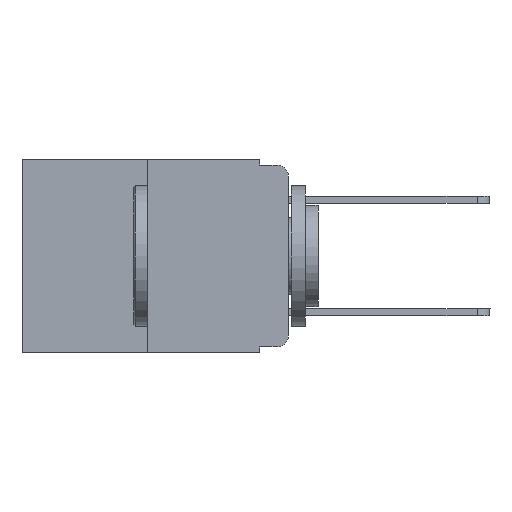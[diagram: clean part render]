
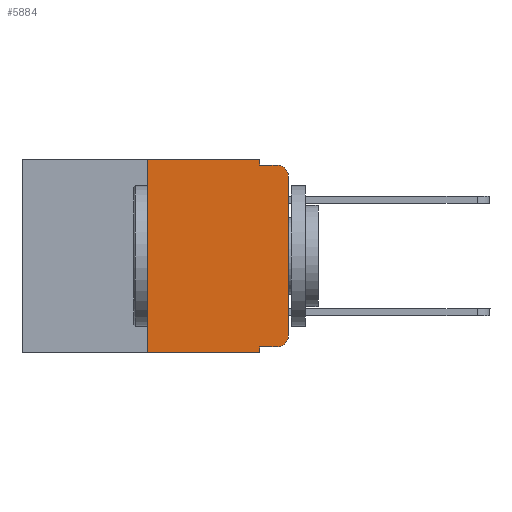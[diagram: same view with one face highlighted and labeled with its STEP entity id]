
A CAD part, left-side view. The second image highlights one B-rep face of the part: STEP entity #5884.
In plain terms, the highlighted planar face has unit normal (-1, 0, 0).
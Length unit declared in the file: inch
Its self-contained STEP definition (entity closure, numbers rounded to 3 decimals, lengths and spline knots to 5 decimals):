
#349 = CARTESIAN_POINT ( 'NONE',  ( 0., 0.051, -0.333 ) ) ;
#657 = DIRECTION ( 'NONE',  ( 0., -1., 0. ) ) ;
#759 = CARTESIAN_POINT ( 'NONE',  ( 0., 0.051, 0. ) ) ;
#1233 = LINE ( 'NONE', #5460, #2281 ) ;
#1268 = CARTESIAN_POINT ( 'NONE',  ( 0., 0.473, 0. ) ) ;
#1450 = LINE ( 'NONE', #349, #11938 ) ;
#1746 = CARTESIAN_POINT ( 'NONE',  ( 0., 0.051, -0.01 ) ) ;
#2281 = VECTOR ( 'NONE', #13563, 39.37008 ) ;
#2683 = ORIENTED_EDGE ( 'NONE', *, *, #13855, .F. ) ;
#2717 = EDGE_CURVE ( 'NONE', #15281, #13581, #4528, .T. ) ;
#2889 = DIRECTION ( 'NONE',  ( 1., 0., 0. ) ) ;
#2960 = DIRECTION ( 'NONE',  ( 0., -1., 0. ) ) ;
#2986 = VERTEX_POINT ( 'NONE', #11267 ) ;
#2997 = EDGE_CURVE ( 'NONE', #15556, #3769, #9913, .T. ) ;
#3769 = VERTEX_POINT ( 'NONE', #13083 ) ;
#3792 = DIRECTION ( 'NONE',  ( -1., 0., 0. ) ) ;
#4029 = EDGE_CURVE ( 'NONE', #12999, #17252, #9879, .T. ) ;
#4117 = DIRECTION ( 'NONE',  ( 0., 0., -1. ) ) ;
#4300 = VECTOR ( 'NONE', #4349, 39.37008 ) ;
#4349 = DIRECTION ( 'NONE',  ( 0., -1., 0. ) ) ;
#4528 = LINE ( 'NONE', #1268, #10793 ) ;
#4591 = ORIENTED_EDGE ( 'NONE', *, *, #5762, .T. ) ;
#4881 = CARTESIAN_POINT ( 'NONE',  ( 0., 0.02, -0.333 ) ) ;
#5241 = EDGE_CURVE ( 'NONE', #2986, #13518, #1450, .T. ) ;
#5460 = CARTESIAN_POINT ( 'NONE',  ( 0., 0.25, 0. ) ) ;
#5762 = EDGE_CURVE ( 'NONE', #13518, #15556, #9610, .T. ) ;
#5884 = ADVANCED_FACE ( 'NONE', ( #13840 ), #8219, .F. ) ;
#6357 = DIRECTION ( 'NONE',  ( 0., 0., -1. ) ) ;
#6586 = ORIENTED_EDGE ( 'NONE', *, *, #2717, .F. ) ;
#6809 = EDGE_CURVE ( 'NONE', #2986, #10002, #9360, .T. ) ;
#6993 = VECTOR ( 'NONE', #6357, 39.37008 ) ;
#7053 = CARTESIAN_POINT ( 'NONE',  ( 0., 0.02, -0.313 ) ) ;
#7105 = DIRECTION ( 'NONE',  ( 0., 0., 1. ) ) ;
#7836 = ORIENTED_EDGE ( 'NONE', *, *, #2997, .T. ) ;
#7860 = AXIS2_PLACEMENT_3D ( 'NONE', #10647, #3792, #13372 ) ;
#7878 = EDGE_CURVE ( 'NONE', #13581, #12999, #11845, .T. ) ;
#8146 = DIRECTION ( 'NONE',  ( 0., -1., 0. ) ) ;
#8163 = DIRECTION ( 'NONE',  ( -1., 0., 0. ) ) ;
#8210 = ORIENTED_EDGE ( 'NONE', *, *, #10083, .T. ) ;
#8219 = PLANE ( 'NONE',  #8493 ) ;
#8387 = CARTESIAN_POINT ( 'NONE',  ( 0., 0., -0.313 ) ) ;
#8493 = AXIS2_PLACEMENT_3D ( 'NONE', #11113, #2889, #12490 ) ;
#8900 = CARTESIAN_POINT ( 'NONE',  ( 0., 0.473, -0.343 ) ) ;
#9342 = VERTEX_POINT ( 'NONE', #14254 ) ;
#9360 = LINE ( 'NONE', #759, #6993 ) ;
#9529 = LINE ( 'NONE', #8900, #15245 ) ;
#9610 = CIRCLE ( 'NONE', #17261, 0.02 ) ;
#9637 = ORIENTED_EDGE ( 'NONE', *, *, #7878, .F. ) ;
#9658 = EDGE_CURVE ( 'NONE', #9342, #10002, #9529, .T. ) ;
#9879 = LINE ( 'NONE', #1746, #4300 ) ;
#9913 = LINE ( 'NONE', #10078, #12883 ) ;
#10002 = VERTEX_POINT ( 'NONE', #11820 ) ;
#10078 = CARTESIAN_POINT ( 'NONE',  ( 0., 0., 0. ) ) ;
#10083 = EDGE_CURVE ( 'NONE', #3769, #17252, #11199, .T. ) ;
#10469 = CARTESIAN_POINT ( 'NONE',  ( 0., 0.051, 0. ) ) ;
#10647 = CARTESIAN_POINT ( 'NONE',  ( 0., 0.02, -0.03 ) ) ;
#10793 = VECTOR ( 'NONE', #8146, 39.37008 ) ;
#11113 = CARTESIAN_POINT ( 'NONE',  ( 0., 0.473, 0. ) ) ;
#11199 = CIRCLE ( 'NONE', #7860, 0.02 ) ;
#11267 = CARTESIAN_POINT ( 'NONE',  ( 0., 0.051, -0.333 ) ) ;
#11652 = CARTESIAN_POINT ( 'NONE',  ( 0., 0.25, 0. ) ) ;
#11820 = CARTESIAN_POINT ( 'NONE',  ( 0., 0.051, -0.343 ) ) ;
#11845 = LINE ( 'NONE', #10469, #15883 ) ;
#11938 = VECTOR ( 'NONE', #2960, 39.37008 ) ;
#12274 = CARTESIAN_POINT ( 'NONE',  ( 0., 0.02, -0.01 ) ) ;
#12490 = DIRECTION ( 'NONE',  ( 0., 0., -1. ) ) ;
#12883 = VECTOR ( 'NONE', #7105, 39.37008 ) ;
#12999 = VERTEX_POINT ( 'NONE', #16195 ) ;
#13015 = CARTESIAN_POINT ( 'NONE',  ( 0., 0.051, 0. ) ) ;
#13083 = CARTESIAN_POINT ( 'NONE',  ( 0., 0., -0.03 ) ) ;
#13372 = DIRECTION ( 'NONE',  ( 0., 0., -1. ) ) ;
#13518 = VERTEX_POINT ( 'NONE', #4881 ) ;
#13563 = DIRECTION ( 'NONE',  ( 0., 0., 1. ) ) ;
#13581 = VERTEX_POINT ( 'NONE', #13015 ) ;
#13840 = FACE_OUTER_BOUND ( 'NONE', #15627, .T. ) ;
#13855 = EDGE_CURVE ( 'NONE', #9342, #15281, #1233, .T. ) ;
#14254 = CARTESIAN_POINT ( 'NONE',  ( 0., 0.25, -0.343 ) ) ;
#14563 = DIRECTION ( 'NONE',  ( 0., 0., -1. ) ) ;
#14641 = ORIENTED_EDGE ( 'NONE', *, *, #9658, .T. ) ;
#14799 = ORIENTED_EDGE ( 'NONE', *, *, #6809, .F. ) ;
#15245 = VECTOR ( 'NONE', #657, 39.37008 ) ;
#15281 = VERTEX_POINT ( 'NONE', #11652 ) ;
#15314 = ORIENTED_EDGE ( 'NONE', *, *, #5241, .T. ) ;
#15556 = VERTEX_POINT ( 'NONE', #8387 ) ;
#15627 = EDGE_LOOP ( 'NONE', ( #7836, #8210, #16170, #9637, #6586, #2683, #14641, #14799, #15314, #4591 ) ) ;
#15883 = VECTOR ( 'NONE', #14563, 39.37008 ) ;
#16170 = ORIENTED_EDGE ( 'NONE', *, *, #4029, .F. ) ;
#16195 = CARTESIAN_POINT ( 'NONE',  ( 0., 0.051, -0.01 ) ) ;
#17252 = VERTEX_POINT ( 'NONE', #12274 ) ;
#17261 = AXIS2_PLACEMENT_3D ( 'NONE', #7053, #8163, #4117 ) ;
